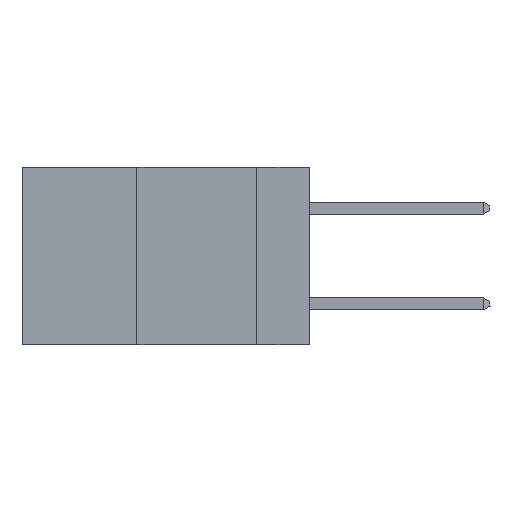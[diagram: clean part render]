
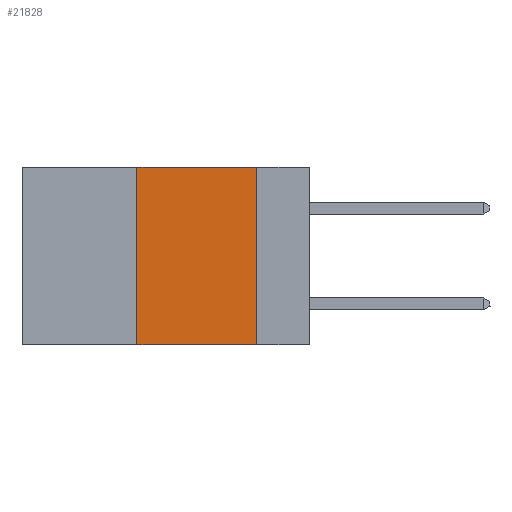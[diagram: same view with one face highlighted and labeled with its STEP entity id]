
A CAD part, left-side view. The second image highlights one B-rep face of the part: STEP entity #21828.
In plain terms, the highlighted planar face has unit normal (-1, 0, 0).
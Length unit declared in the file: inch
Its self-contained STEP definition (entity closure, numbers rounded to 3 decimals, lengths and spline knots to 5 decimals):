
#147 = DIRECTION ( 'NONE',  ( 1., 0., 0. ) ) ;
#2559 = CARTESIAN_POINT ( 'NONE',  ( 0., 0.11, 0. ) ) ;
#2650 = EDGE_CURVE ( 'NONE', #4335, #16295, #10580, .T. ) ;
#3468 = VECTOR ( 'NONE', #6938, 39.37008 ) ;
#4084 = CARTESIAN_POINT ( 'NONE',  ( 0., 0.11, -0.37 ) ) ;
#4335 = VERTEX_POINT ( 'NONE', #15487 ) ;
#5293 = LINE ( 'NONE', #12471, #17622 ) ;
#6938 = DIRECTION ( 'NONE',  ( 0., -1., 0. ) ) ;
#7125 = LINE ( 'NONE', #18028, #11092 ) ;
#8537 = ORIENTED_EDGE ( 'NONE', *, *, #16655, .F. ) ;
#8593 = FACE_OUTER_BOUND ( 'NONE', #17873, .T. ) ;
#8907 = CARTESIAN_POINT ( 'NONE',  ( 0., 0.11, 0. ) ) ;
#8910 = ORIENTED_EDGE ( 'NONE', *, *, #9174, .F. ) ;
#9174 = EDGE_CURVE ( 'NONE', #14858, #22231, #7125, .T. ) ;
#9718 = DIRECTION ( 'NONE',  ( 0., 0., -1. ) ) ;
#9822 = LINE ( 'NONE', #2559, #16678 ) ;
#10580 = LINE ( 'NONE', #19620, #3468 ) ;
#11092 = VECTOR ( 'NONE', #17785, 39.37008 ) ;
#11672 = ORIENTED_EDGE ( 'NONE', *, *, #2650, .T. ) ;
#12340 = CARTESIAN_POINT ( 'NONE',  ( 0., 0.6, 0. ) ) ;
#12471 = CARTESIAN_POINT ( 'NONE',  ( 0., 0.36, 0. ) ) ;
#14723 = ORIENTED_EDGE ( 'NONE', *, *, #22513, .F. ) ;
#14858 = VERTEX_POINT ( 'NONE', #19660 ) ;
#15487 = CARTESIAN_POINT ( 'NONE',  ( 0., 0.36, -0.37 ) ) ;
#15735 = DIRECTION ( 'NONE',  ( 0., 0., -1. ) ) ;
#16295 = VERTEX_POINT ( 'NONE', #4084 ) ;
#16655 = EDGE_CURVE ( 'NONE', #4335, #14858, #5293, .T. ) ;
#16678 = VECTOR ( 'NONE', #9718, 39.37008 ) ;
#17622 = VECTOR ( 'NONE', #19631, 39.37008 ) ;
#17785 = DIRECTION ( 'NONE',  ( 0., -1., 0. ) ) ;
#17873 = EDGE_LOOP ( 'NONE', ( #14723, #8910, #8537, #11672 ) ) ;
#18028 = CARTESIAN_POINT ( 'NONE',  ( 0., 0.6, 0. ) ) ;
#19620 = CARTESIAN_POINT ( 'NONE',  ( 0., 0.6, -0.37 ) ) ;
#19631 = DIRECTION ( 'NONE',  ( 0., 0., 1. ) ) ;
#19660 = CARTESIAN_POINT ( 'NONE',  ( 0., 0.36, 0. ) ) ;
#21167 = AXIS2_PLACEMENT_3D ( 'NONE', #12340, #147, #15735 ) ;
#21374 = PLANE ( 'NONE',  #21167 ) ;
#21828 = ADVANCED_FACE ( 'NONE', ( #8593 ), #21374, .F. ) ;
#22231 = VERTEX_POINT ( 'NONE', #8907 ) ;
#22513 = EDGE_CURVE ( 'NONE', #22231, #16295, #9822, .T. ) ;
